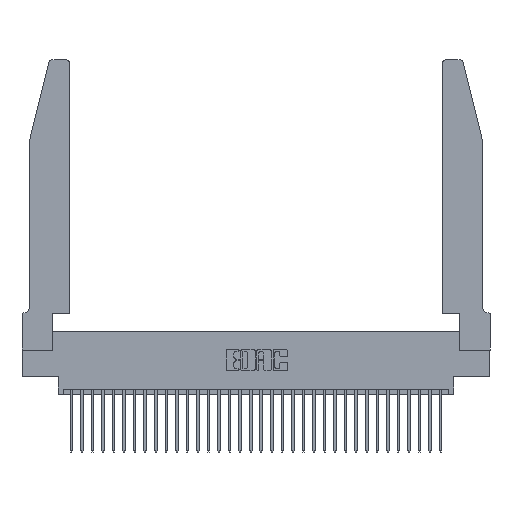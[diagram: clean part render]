
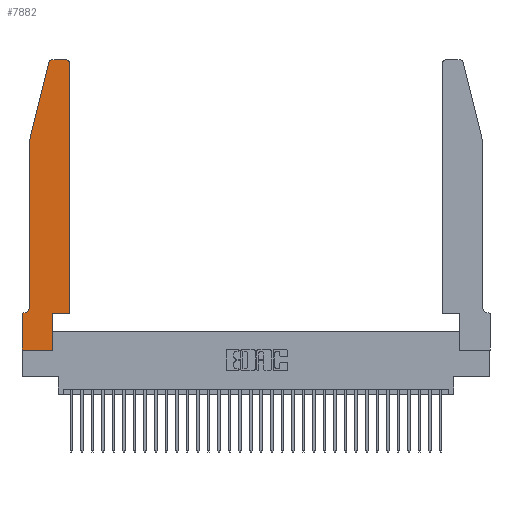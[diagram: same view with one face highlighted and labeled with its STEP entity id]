
A CAD part, top view. The second image highlights one B-rep face of the part: STEP entity #7882.
In plain terms, the highlighted planar face has unit normal (0, 0, 1).
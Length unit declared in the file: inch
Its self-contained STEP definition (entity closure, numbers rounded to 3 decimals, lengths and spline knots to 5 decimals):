
#426 = VERTEX_POINT ( 'NONE', #11715 ) ;
#457 = DIRECTION ( 'NONE',  ( 0., 0., -1. ) ) ;
#1002 = DIRECTION ( 'NONE',  ( 1., 0., 0. ) ) ;
#1386 = VECTOR ( 'NONE', #4601, 39.37008 ) ;
#1630 = VECTOR ( 'NONE', #18039, 39.37008 ) ;
#1852 = DIRECTION ( 'NONE',  ( 0., -1., 0. ) ) ;
#1861 = CARTESIAN_POINT ( 'NONE',  ( 0.2605, 2.75, 0.37 ) ) ;
#1948 = CIRCLE ( 'NONE', #7091, 0.07 ) ;
#2020 = VECTOR ( 'NONE', #1852, 39.37008 ) ;
#3150 = EDGE_CURVE ( 'NONE', #13368, #9378, #14671, .T. ) ;
#3609 = CARTESIAN_POINT ( 'NONE',  ( 0.4505, 0.35, 0.37 ) ) ;
#3954 = VERTEX_POINT ( 'NONE', #23031 ) ;
#3963 = ORIENTED_EDGE ( 'NONE', *, *, #15289, .T. ) ;
#4090 = DIRECTION ( 'NONE',  ( 1., 0., 0. ) ) ;
#4171 = VECTOR ( 'NONE', #17706, 39.37008 ) ;
#4601 = DIRECTION ( 'NONE',  ( -1., 0., 0. ) ) ;
#4956 = CARTESIAN_POINT ( 'NONE',  ( 0., 0., 0.37 ) ) ;
#6279 = VERTEX_POINT ( 'NONE', #29062 ) ;
#6423 = CIRCLE ( 'NONE', #16794, 0.03 ) ;
#6560 = DIRECTION ( 'NONE',  ( 0., 1., 0. ) ) ;
#6924 = DIRECTION ( 'NONE',  ( 0., 0., 1. ) ) ;
#7044 = EDGE_CURVE ( 'NONE', #6279, #3954, #1948, .T. ) ;
#7091 = AXIS2_PLACEMENT_3D ( 'NONE', #16460, #457, #19043 ) ;
#7882 = ADVANCED_FACE ( 'NONE', ( #13268 ), #32757, .T. ) ;
#8286 = DIRECTION ( 'NONE',  ( 1., 0., 0. ) ) ;
#8843 = LINE ( 'NONE', #23109, #1630 ) ;
#9244 = EDGE_CURVE ( 'NONE', #11848, #426, #22471, .T. ) ;
#9378 = VERTEX_POINT ( 'NONE', #4956 ) ;
#9624 = DIRECTION ( 'NONE',  ( -1., 0., 0. ) ) ;
#9903 = VERTEX_POINT ( 'NONE', #17856 ) ;
#10507 = CARTESIAN_POINT ( 'NONE',  ( 0.25487, 2.72718, 0.37 ) ) ;
#11135 = ORIENTED_EDGE ( 'NONE', *, *, #30854, .T. ) ;
#11326 = VERTEX_POINT ( 'NONE', #18228 ) ;
#11522 = ORIENTED_EDGE ( 'NONE', *, *, #12073, .T. ) ;
#11715 = CARTESIAN_POINT ( 'NONE',  ( 0.284, 2.75, 0.37 ) ) ;
#11848 = VERTEX_POINT ( 'NONE', #23025 ) ;
#11877 = CARTESIAN_POINT ( 'NONE',  ( 0.4505, 0.35, 0.37 ) ) ;
#12073 = EDGE_CURVE ( 'NONE', #27614, #6279, #22279, .T. ) ;
#12784 = ORIENTED_EDGE ( 'NONE', *, *, #29749, .T. ) ;
#13055 = VECTOR ( 'NONE', #14527, 39.37008 ) ;
#13268 = FACE_OUTER_BOUND ( 'NONE', #26052, .T. ) ;
#13368 = VERTEX_POINT ( 'NONE', #18032 ) ;
#14283 = CIRCLE ( 'NONE', #30088, 0.03 ) ;
#14423 = EDGE_CURVE ( 'NONE', #9903, #11848, #14283, .T. ) ;
#14527 = DIRECTION ( 'NONE',  ( 1., 0., 0. ) ) ;
#14671 = LINE ( 'NONE', #30033, #21533 ) ;
#14825 = ORIENTED_EDGE ( 'NONE', *, *, #23619, .T. ) ;
#15120 = CARTESIAN_POINT ( 'NONE',  ( 0.0755, 2., 0.37 ) ) ;
#15189 = CARTESIAN_POINT ( 'NONE',  ( 0.0755, 2., 0.37 ) ) ;
#15289 = EDGE_CURVE ( 'NONE', #11326, #16028, #8843, .T. ) ;
#16029 = ORIENTED_EDGE ( 'NONE', *, *, #9244, .T. ) ;
#16028 = VERTEX_POINT ( 'NONE', #23859 ) ;
#16285 = LINE ( 'NONE', #23887, #23932 ) ;
#16460 = CARTESIAN_POINT ( 'NONE',  ( 0.0055, 0.42, 0.37 ) ) ;
#16794 = AXIS2_PLACEMENT_3D ( 'NONE', #32393, #16968, #1002 ) ;
#16968 = DIRECTION ( 'NONE',  ( 0., 0., 1. ) ) ;
#17231 = DIRECTION ( 'NONE',  ( 0., -1., 0. ) ) ;
#17249 = ORIENTED_EDGE ( 'NONE', *, *, #23123, .T. ) ;
#17311 = CARTESIAN_POINT ( 'NONE',  ( 0., 0.35, 0.37 ) ) ;
#17633 = ORIENTED_EDGE ( 'NONE', *, *, #32362, .T. ) ;
#17706 = DIRECTION ( 'NONE',  ( -0.239, -0.971, 0. ) ) ;
#17856 = CARTESIAN_POINT ( 'NONE',  ( 0.4505, 2.72, 0.37 ) ) ;
#18032 = CARTESIAN_POINT ( 'NONE',  ( 0., 0.35, 0.37 ) ) ;
#18039 = DIRECTION ( 'NONE',  ( 0., 1., 0. ) ) ;
#18228 = CARTESIAN_POINT ( 'NONE',  ( 0.2865, 0., 0.37 ) ) ;
#18264 = LINE ( 'NONE', #15120, #4171 ) ;
#18794 = LINE ( 'NONE', #3609, #24834 ) ;
#19043 = DIRECTION ( 'NONE',  ( -1., 0., 0. ) ) ;
#19912 = DIRECTION ( 'NONE',  ( 0., 0., 1. ) ) ;
#21494 = LINE ( 'NONE', #25176, #22294 ) ;
#21533 = VECTOR ( 'NONE', #17231, 39.37008 ) ;
#22279 = LINE ( 'NONE', #15189, #2020 ) ;
#22294 = VECTOR ( 'NONE', #9624, 39.37008 ) ;
#22471 = LINE ( 'NONE', #1861, #1386 ) ;
#22599 = CARTESIAN_POINT ( 'NONE',  ( 0.4205, 2.72, 0.37 ) ) ;
#23025 = CARTESIAN_POINT ( 'NONE',  ( 0.4205, 2.75, 0.37 ) ) ;
#23031 = CARTESIAN_POINT ( 'NONE',  ( 0.0055, 0.35, 0.37 ) ) ;
#23109 = CARTESIAN_POINT ( 'NONE',  ( 0.2865, 0.35, 0.37 ) ) ;
#23123 = EDGE_CURVE ( 'NONE', #9378, #11326, #16285, .T. ) ;
#23619 = EDGE_CURVE ( 'NONE', #3954, #13368, #21494, .T. ) ;
#23749 = CARTESIAN_POINT ( 'NONE',  ( 0.0755, 2., 0.37 ) ) ;
#23859 = CARTESIAN_POINT ( 'NONE',  ( 0.2865, 0.35, 0.37 ) ) ;
#23887 = CARTESIAN_POINT ( 'NONE',  ( 0., 0., 0.37 ) ) ;
#23932 = VECTOR ( 'NONE', #8286, 39.37008 ) ;
#24834 = VECTOR ( 'NONE', #6560, 39.37008 ) ;
#25040 = AXIS2_PLACEMENT_3D ( 'NONE', #17311, #19912, #4090 ) ;
#25176 = CARTESIAN_POINT ( 'NONE',  ( 0.0755, 0.35, 0.37 ) ) ;
#25196 = DIRECTION ( 'NONE',  ( 1., 0., 0. ) ) ;
#26052 = EDGE_LOOP ( 'NONE', ( #16029, #29679, #17633, #11522, #26103, #14825, #28493, #17249, #3963, #11135, #12784, #33400 ) ) ;
#26103 = ORIENTED_EDGE ( 'NONE', *, *, #7044, .T. ) ;
#26768 = CARTESIAN_POINT ( 'NONE',  ( 0.4505, 0.35, 0.37 ) ) ;
#27521 = VERTEX_POINT ( 'NONE', #10507 ) ;
#27565 = LINE ( 'NONE', #11877, #13055 ) ;
#27614 = VERTEX_POINT ( 'NONE', #23749 ) ;
#28493 = ORIENTED_EDGE ( 'NONE', *, *, #3150, .T. ) ;
#29062 = CARTESIAN_POINT ( 'NONE',  ( 0.0755, 0.42, 0.37 ) ) ;
#29581 = VERTEX_POINT ( 'NONE', #26768 ) ;
#29679 = ORIENTED_EDGE ( 'NONE', *, *, #29705, .T. ) ;
#29705 = EDGE_CURVE ( 'NONE', #426, #27521, #6423, .T. ) ;
#29749 = EDGE_CURVE ( 'NONE', #29581, #9903, #18794, .T. ) ;
#30033 = CARTESIAN_POINT ( 'NONE',  ( 0., 0., 0.37 ) ) ;
#30088 = AXIS2_PLACEMENT_3D ( 'NONE', #22599, #6924, #25196 ) ;
#30854 = EDGE_CURVE ( 'NONE', #16028, #29581, #27565, .T. ) ;
#32362 = EDGE_CURVE ( 'NONE', #27521, #27614, #18264, .T. ) ;
#32393 = CARTESIAN_POINT ( 'NONE',  ( 0.284, 2.72, 0.37 ) ) ;
#32757 = PLANE ( 'NONE',  #25040 ) ;
#33400 = ORIENTED_EDGE ( 'NONE', *, *, #14423, .T. ) ;
